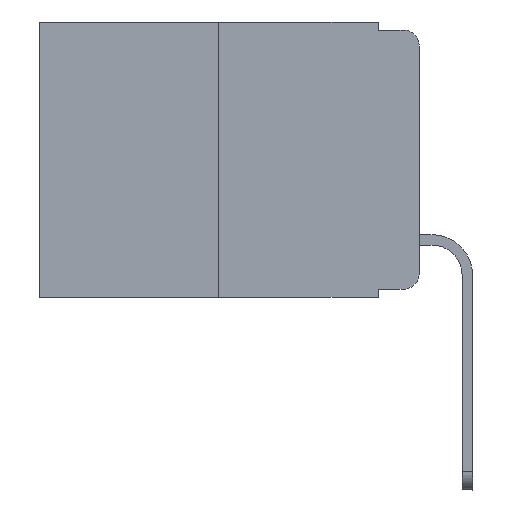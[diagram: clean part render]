
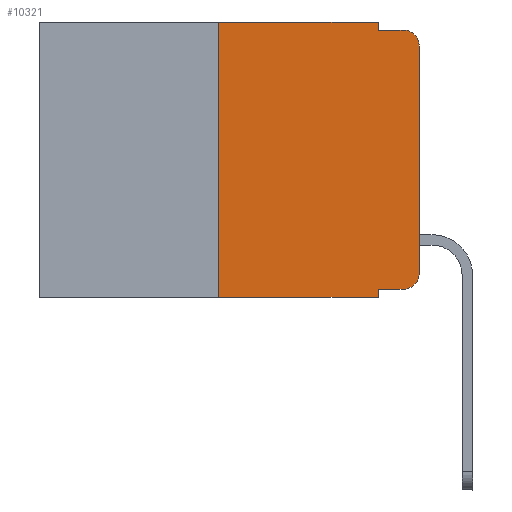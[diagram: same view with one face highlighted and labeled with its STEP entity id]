
A CAD part, left-side view. The second image highlights one B-rep face of the part: STEP entity #10321.
In plain terms, the highlighted planar face has unit normal (-1, 0, 0).
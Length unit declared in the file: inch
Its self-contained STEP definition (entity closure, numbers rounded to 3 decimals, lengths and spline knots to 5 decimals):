
#87 = CARTESIAN_POINT ( 'NONE',  ( 0., 0.02, -0.01 ) ) ;
#268 = VECTOR ( 'NONE', #4491, 39.37008 ) ;
#395 = LINE ( 'NONE', #7064, #8637 ) ;
#441 = VECTOR ( 'NONE', #5893, 39.37008 ) ;
#596 = EDGE_CURVE ( 'NONE', #5351, #3482, #2389, .T. ) ;
#709 = AXIS2_PLACEMENT_3D ( 'NONE', #822, #2434, #5829 ) ;
#719 = CARTESIAN_POINT ( 'NONE',  ( 0., 0.051, -0.01 ) ) ;
#765 = ORIENTED_EDGE ( 'NONE', *, *, #5180, .T. ) ;
#822 = CARTESIAN_POINT ( 'NONE',  ( 0., 0.02, -0.313 ) ) ;
#996 = DIRECTION ( 'NONE',  ( 0., 0., 1. ) ) ;
#1023 = VECTOR ( 'NONE', #3168, 39.37008 ) ;
#1077 = LINE ( 'NONE', #9199, #441 ) ;
#1237 = DIRECTION ( 'NONE',  ( 0., 0., -1. ) ) ;
#1374 = ORIENTED_EDGE ( 'NONE', *, *, #3734, .T. ) ;
#1389 = EDGE_CURVE ( 'NONE', #8507, #2507, #6837, .T. ) ;
#1885 = ORIENTED_EDGE ( 'NONE', *, *, #596, .F. ) ;
#2152 = CARTESIAN_POINT ( 'NONE',  ( 0., 0.051, -0.333 ) ) ;
#2241 = LINE ( 'NONE', #719, #268 ) ;
#2249 = DIRECTION ( 'NONE',  ( -1., 0., 0. ) ) ;
#2389 = LINE ( 'NONE', #5674, #3656 ) ;
#2434 = DIRECTION ( 'NONE',  ( -1., 0., 0. ) ) ;
#2507 = VERTEX_POINT ( 'NONE', #87 ) ;
#2546 = VERTEX_POINT ( 'NONE', #2152 ) ;
#2621 = CARTESIAN_POINT ( 'NONE',  ( 0., 0., 0. ) ) ;
#2807 = EDGE_CURVE ( 'NONE', #2546, #9315, #1077, .T. ) ;
#2867 = ORIENTED_EDGE ( 'NONE', *, *, #2966, .F. ) ;
#2876 = VERTEX_POINT ( 'NONE', #5993 ) ;
#2966 = EDGE_CURVE ( 'NONE', #5073, #2507, #2241, .T. ) ;
#3113 = DIRECTION ( 'NONE',  ( 0., 0., -1. ) ) ;
#3168 = DIRECTION ( 'NONE',  ( 0., -1., 0. ) ) ;
#3482 = VERTEX_POINT ( 'NONE', #6874 ) ;
#3559 = ORIENTED_EDGE ( 'NONE', *, *, #7056, .F. ) ;
#3576 = LINE ( 'NONE', #2621, #7227 ) ;
#3609 = LINE ( 'NONE', #3763, #9081 ) ;
#3653 = CARTESIAN_POINT ( 'NONE',  ( 0., 0.473, 0. ) ) ;
#3656 = VECTOR ( 'NONE', #8834, 39.37008 ) ;
#3734 = EDGE_CURVE ( 'NONE', #5484, #8507, #3576, .T. ) ;
#3763 = CARTESIAN_POINT ( 'NONE',  ( 0., 0.051, -0.333 ) ) ;
#4123 = ORIENTED_EDGE ( 'NONE', *, *, #9937, .T. ) ;
#4236 = CARTESIAN_POINT ( 'NONE',  ( 0., 0.051, -0.01 ) ) ;
#4442 = DIRECTION ( 'NONE',  ( 0., -1., 0. ) ) ;
#4491 = DIRECTION ( 'NONE',  ( 0., -1., 0. ) ) ;
#4685 = PLANE ( 'NONE',  #4922 ) ;
#4922 = AXIS2_PLACEMENT_3D ( 'NONE', #3653, #10032, #1237 ) ;
#5073 = VERTEX_POINT ( 'NONE', #4236 ) ;
#5180 = EDGE_CURVE ( 'NONE', #2546, #9863, #3609, .T. ) ;
#5264 = DIRECTION ( 'NONE',  ( 0., -1., 0. ) ) ;
#5351 = VERTEX_POINT ( 'NONE', #10302 ) ;
#5358 = CARTESIAN_POINT ( 'NONE',  ( 0., 0., -0.03 ) ) ;
#5484 = VERTEX_POINT ( 'NONE', #5832 ) ;
#5674 = CARTESIAN_POINT ( 'NONE',  ( 0., 0.25, 0. ) ) ;
#5690 = DIRECTION ( 'NONE',  ( 0., 0., -1. ) ) ;
#5829 = DIRECTION ( 'NONE',  ( 0., 0., -1. ) ) ;
#5832 = CARTESIAN_POINT ( 'NONE',  ( 0., 0., -0.313 ) ) ;
#5893 = DIRECTION ( 'NONE',  ( 0., 0., -1. ) ) ;
#5993 = CARTESIAN_POINT ( 'NONE',  ( 0., 0.051, 0. ) ) ;
#6364 = CARTESIAN_POINT ( 'NONE',  ( 0., 0.473, 0. ) ) ;
#6621 = ORIENTED_EDGE ( 'NONE', *, *, #8253, .F. ) ;
#6673 = AXIS2_PLACEMENT_3D ( 'NONE', #9481, #2249, #5690 ) ;
#6747 = VECTOR ( 'NONE', #3113, 39.37008 ) ;
#6837 = CIRCLE ( 'NONE', #6673, 0.02 ) ;
#6874 = CARTESIAN_POINT ( 'NONE',  ( 0., 0.25, 0. ) ) ;
#7056 = EDGE_CURVE ( 'NONE', #2876, #5073, #8780, .T. ) ;
#7064 = CARTESIAN_POINT ( 'NONE',  ( 0., 0.473, -0.343 ) ) ;
#7208 = LINE ( 'NONE', #6364, #1023 ) ;
#7227 = VECTOR ( 'NONE', #996, 39.37008 ) ;
#8253 = EDGE_CURVE ( 'NONE', #3482, #2876, #7208, .T. ) ;
#8441 = CARTESIAN_POINT ( 'NONE',  ( 0., 0.051, -0.343 ) ) ;
#8507 = VERTEX_POINT ( 'NONE', #5358 ) ;
#8637 = VECTOR ( 'NONE', #5264, 39.37008 ) ;
#8675 = EDGE_CURVE ( 'NONE', #9863, #5484, #9462, .T. ) ;
#8780 = LINE ( 'NONE', #10437, #6747 ) ;
#8834 = DIRECTION ( 'NONE',  ( 0., 0., 1. ) ) ;
#9081 = VECTOR ( 'NONE', #4442, 39.37008 ) ;
#9192 = ORIENTED_EDGE ( 'NONE', *, *, #2807, .F. ) ;
#9199 = CARTESIAN_POINT ( 'NONE',  ( 0., 0.051, 0. ) ) ;
#9228 = ORIENTED_EDGE ( 'NONE', *, *, #8675, .T. ) ;
#9315 = VERTEX_POINT ( 'NONE', #8441 ) ;
#9338 = EDGE_LOOP ( 'NONE', ( #1374, #9739, #2867, #3559, #6621, #1885, #4123, #9192, #765, #9228 ) ) ;
#9462 = CIRCLE ( 'NONE', #709, 0.02 ) ;
#9481 = CARTESIAN_POINT ( 'NONE',  ( 0., 0.02, -0.03 ) ) ;
#9563 = FACE_OUTER_BOUND ( 'NONE', #9338, .T. ) ;
#9739 = ORIENTED_EDGE ( 'NONE', *, *, #1389, .T. ) ;
#9863 = VERTEX_POINT ( 'NONE', #10148 ) ;
#9937 = EDGE_CURVE ( 'NONE', #5351, #9315, #395, .T. ) ;
#10032 = DIRECTION ( 'NONE',  ( 1., 0., 0. ) ) ;
#10148 = CARTESIAN_POINT ( 'NONE',  ( 0., 0.02, -0.333 ) ) ;
#10302 = CARTESIAN_POINT ( 'NONE',  ( 0., 0.25, -0.343 ) ) ;
#10321 = ADVANCED_FACE ( 'NONE', ( #9563 ), #4685, .F. ) ;
#10437 = CARTESIAN_POINT ( 'NONE',  ( 0., 0.051, 0. ) ) ;
